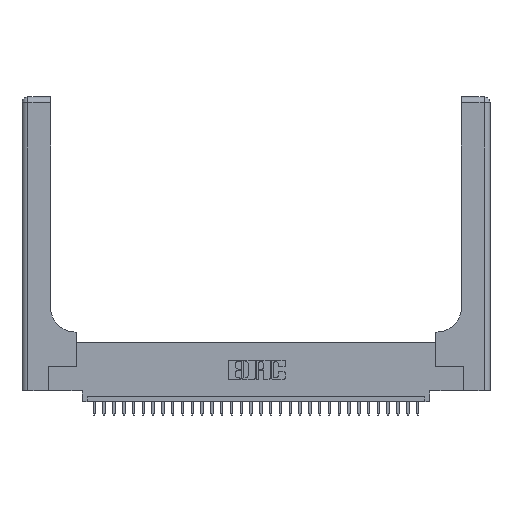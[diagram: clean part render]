
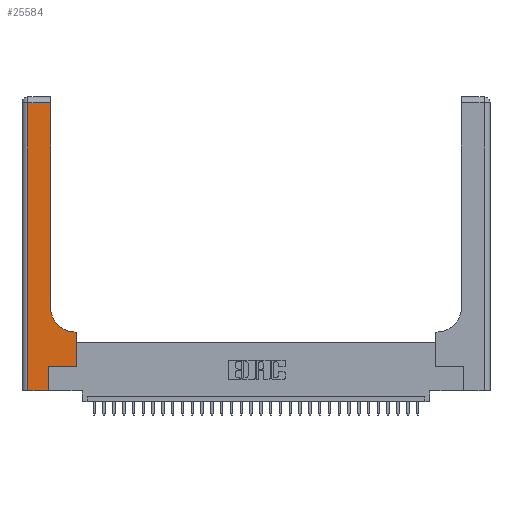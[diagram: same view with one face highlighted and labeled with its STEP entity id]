
A CAD part, top view. The second image highlights one B-rep face of the part: STEP entity #25584.
In plain terms, the highlighted planar face has unit normal (0, 0, 1).
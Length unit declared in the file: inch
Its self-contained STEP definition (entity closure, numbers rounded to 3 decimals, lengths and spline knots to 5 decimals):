
#1242 = CARTESIAN_POINT ( 'NONE',  ( 0.269, 0.25, 0.37 ) ) ;
#1351 = VERTEX_POINT ( 'NONE', #23048 ) ;
#1455 = DIRECTION ( 'NONE',  ( 0., 1., 0. ) ) ;
#2443 = VECTOR ( 'NONE', #18612, 39.37008 ) ;
#3131 = LINE ( 'NONE', #27467, #20122 ) ;
#3362 = ORIENTED_EDGE ( 'NONE', *, *, #4004, .T. ) ;
#4004 = EDGE_CURVE ( 'NONE', #1351, #6792, #24444, .T. ) ;
#4568 = EDGE_CURVE ( 'NONE', #28475, #1351, #25941, .T. ) ;
#4979 = DIRECTION ( 'NONE',  ( 0., 0., -1. ) ) ;
#5131 = CARTESIAN_POINT ( 'NONE',  ( 0.269, 0., 0.37 ) ) ;
#5593 = EDGE_CURVE ( 'NONE', #10277, #28475, #28785, .T. ) ;
#5920 = LINE ( 'NONE', #26173, #2443 ) ;
#6251 = VECTOR ( 'NONE', #16272, 39.37008 ) ;
#6440 = VERTEX_POINT ( 'NONE', #26564 ) ;
#6703 = CARTESIAN_POINT ( 'NONE',  ( 0.06, 2.94, 0.37 ) ) ;
#6774 = EDGE_CURVE ( 'NONE', #6792, #24310, #22166, .T. ) ;
#6776 = EDGE_CURVE ( 'NONE', #15865, #31199, #5920, .T. ) ;
#6792 = VERTEX_POINT ( 'NONE', #18716 ) ;
#6843 = EDGE_CURVE ( 'NONE', #31199, #10277, #27919, .T. ) ;
#7245 = CARTESIAN_POINT ( 'NONE',  ( 0.2915, 2.94, 0.37 ) ) ;
#7382 = FACE_OUTER_BOUND ( 'NONE', #22073, .T. ) ;
#10277 = VERTEX_POINT ( 'NONE', #29114 ) ;
#11203 = EDGE_CURVE ( 'NONE', #24310, #26197, #18737, .T. ) ;
#11615 = ORIENTED_EDGE ( 'NONE', *, *, #4568, .T. ) ;
#12099 = LINE ( 'NONE', #28417, #6251 ) ;
#12367 = CARTESIAN_POINT ( 'NONE',  ( 0., 3., 0.37 ) ) ;
#12474 = PLANE ( 'NONE',  #13188 ) ;
#13188 = AXIS2_PLACEMENT_3D ( 'NONE', #12367, #29475, #17436 ) ;
#13584 = ORIENTED_EDGE ( 'NONE', *, *, #25182, .T. ) ;
#14030 = EDGE_CURVE ( 'NONE', #6440, #15865, #12099, .T. ) ;
#15865 = VERTEX_POINT ( 'NONE', #5131 ) ;
#16272 = DIRECTION ( 'NONE',  ( 1., 0., 0. ) ) ;
#17196 = VECTOR ( 'NONE', #20084, 39.37008 ) ;
#17436 = DIRECTION ( 'NONE',  ( -1., 0., 0. ) ) ;
#17530 = VECTOR ( 'NONE', #1455, 39.37008 ) ;
#17666 = DIRECTION ( 'NONE',  ( 0., -1., 0. ) ) ;
#18612 = DIRECTION ( 'NONE',  ( 0., 1., 0. ) ) ;
#18716 = CARTESIAN_POINT ( 'NONE',  ( 0.2915, 0.85, 0.37 ) ) ;
#18737 = LINE ( 'NONE', #29977, #17196 ) ;
#18834 = CARTESIAN_POINT ( 'NONE',  ( 0.2915, 3., 0.37 ) ) ;
#19464 = CARTESIAN_POINT ( 'NONE',  ( 0.5415, 0.85, 0.37 ) ) ;
#19908 = CARTESIAN_POINT ( 'NONE',  ( 0.5585, 0.25, 0.37 ) ) ;
#20084 = DIRECTION ( 'NONE',  ( -1., 0., 0. ) ) ;
#20122 = VECTOR ( 'NONE', #17666, 39.37008 ) ;
#20232 = VECTOR ( 'NONE', #23590, 39.37008 ) ;
#21567 = AXIS2_PLACEMENT_3D ( 'NONE', #19464, #4979, #24435 ) ;
#22073 = EDGE_LOOP ( 'NONE', ( #28207, #25831, #13584, #23609, #29646, #28093, #22571, #11615, #3362 ) ) ;
#22166 = LINE ( 'NONE', #18834, #17530 ) ;
#22571 = ORIENTED_EDGE ( 'NONE', *, *, #5593, .T. ) ;
#22835 = VECTOR ( 'NONE', #26808, 39.37008 ) ;
#23048 = CARTESIAN_POINT ( 'NONE',  ( 0.5415, 0.6, 0.37 ) ) ;
#23590 = DIRECTION ( 'NONE',  ( 1., 0., 0. ) ) ;
#23609 = ORIENTED_EDGE ( 'NONE', *, *, #14030, .T. ) ;
#23649 = CARTESIAN_POINT ( 'NONE',  ( 0.269, 0.25, 0.37 ) ) ;
#24310 = VERTEX_POINT ( 'NONE', #7245 ) ;
#24349 = CARTESIAN_POINT ( 'NONE',  ( 0.2915, 0.6, 0.37 ) ) ;
#24435 = DIRECTION ( 'NONE',  ( 1., 0., 0. ) ) ;
#24444 = CIRCLE ( 'NONE', #21567, 0.25 ) ;
#24785 = DIRECTION ( 'NONE',  ( 0., 1., 0. ) ) ;
#25182 = EDGE_CURVE ( 'NONE', #26197, #6440, #3131, .T. ) ;
#25505 = CARTESIAN_POINT ( 'NONE',  ( 0.5585, 0.6, 0.37 ) ) ;
#25584 = ADVANCED_FACE ( 'NONE', ( #7382 ), #12474, .F. ) ;
#25831 = ORIENTED_EDGE ( 'NONE', *, *, #11203, .T. ) ;
#25941 = LINE ( 'NONE', #24349, #22835 ) ;
#26173 = CARTESIAN_POINT ( 'NONE',  ( 0.269, 0., 0.37 ) ) ;
#26197 = VERTEX_POINT ( 'NONE', #6703 ) ;
#26564 = CARTESIAN_POINT ( 'NONE',  ( 0.06, 0., 0.37 ) ) ;
#26808 = DIRECTION ( 'NONE',  ( -1., 0., 0. ) ) ;
#27243 = VECTOR ( 'NONE', #24785, 39.37008 ) ;
#27467 = CARTESIAN_POINT ( 'NONE',  ( 0.06, 3., 0.37 ) ) ;
#27919 = LINE ( 'NONE', #1242, #20232 ) ;
#28093 = ORIENTED_EDGE ( 'NONE', *, *, #6843, .T. ) ;
#28207 = ORIENTED_EDGE ( 'NONE', *, *, #6774, .T. ) ;
#28417 = CARTESIAN_POINT ( 'NONE',  ( 0., 0., 0.37 ) ) ;
#28475 = VERTEX_POINT ( 'NONE', #25505 ) ;
#28785 = LINE ( 'NONE', #19908, #27243 ) ;
#29114 = CARTESIAN_POINT ( 'NONE',  ( 0.5585, 0.25, 0.37 ) ) ;
#29475 = DIRECTION ( 'NONE',  ( 0., 0., -1. ) ) ;
#29646 = ORIENTED_EDGE ( 'NONE', *, *, #6776, .T. ) ;
#29977 = CARTESIAN_POINT ( 'NONE',  ( 0., 2.94, 0.37 ) ) ;
#31199 = VERTEX_POINT ( 'NONE', #23649 ) ;
